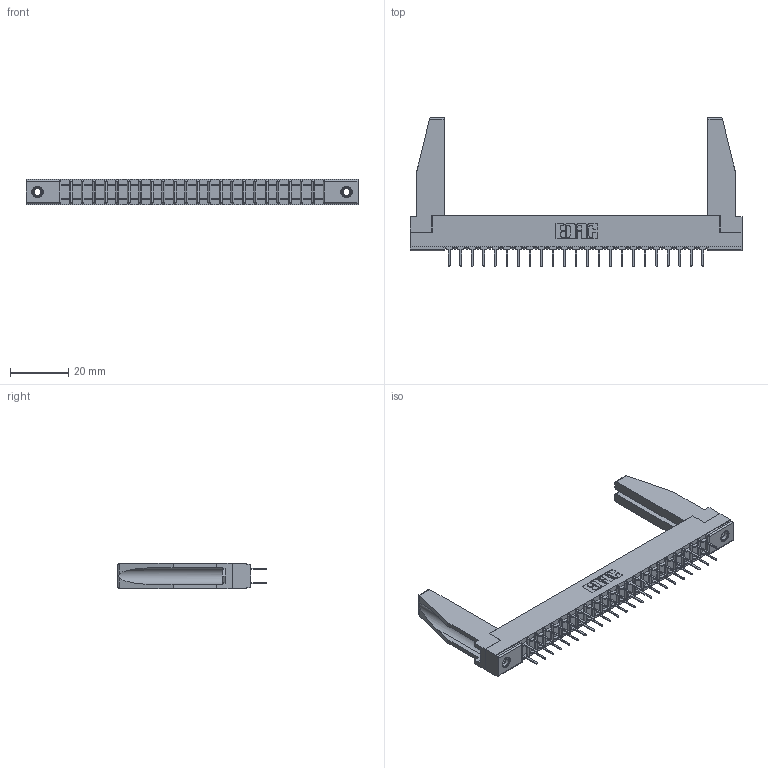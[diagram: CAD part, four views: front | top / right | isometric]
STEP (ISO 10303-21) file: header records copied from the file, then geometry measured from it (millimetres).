
FILE_DESCRIPTION (( 'STEP AP203' ), '1' );
FILE_NAME ('307-046-424-278.STEP', '2020-09-30T02:14:02', ( '' ), ( '' ), 'SwSTEP 2.0', 'SolidWorks 2020', '' );
FILE_SCHEMA (( 'CONFIG_CONTROL_DESIGN' ));
Length unit declared in the file: inch
Products named in the file (5): 307-290-001_524; 307-220-078; 345-250-001_345-250-001-102; 307 Part_.156 Dia Mounting Holes; 307-046-424-278
Assembly tree (51 placements, depth 2):
  307-046-424-278
    307 Part_.156 Dia Mounting Holes
    307-290-001_524  x46
    307-220-078  x2
    345-250-001_345-250-001-102  x2
Bounding box: 114.15 x 51.13 x 8.71 mm (x, y, z)
Volume: 11444.8 mm3; surface area: 16958.9 mm2
Topology: 51 solids, 51 shells, 2388 faces, 6633 edges, 4286 vertices
Faces by surface type: plane 1580, cylinder 744, sphere 48, cone 12, torus 4
Entity records: 25203 total; most frequent: CARTESIAN_POINT 4137, ORIENTED_EDGE 4056, DIRECTION 4014, EDGE_CURVE 2028, VECTOR 1552, LINE 1552, VERTEX_POINT 1312, AXIS2_PLACEMENT_3D 1231
